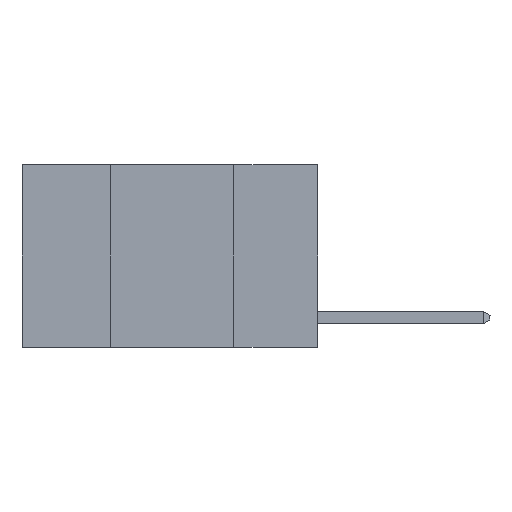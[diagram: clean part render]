
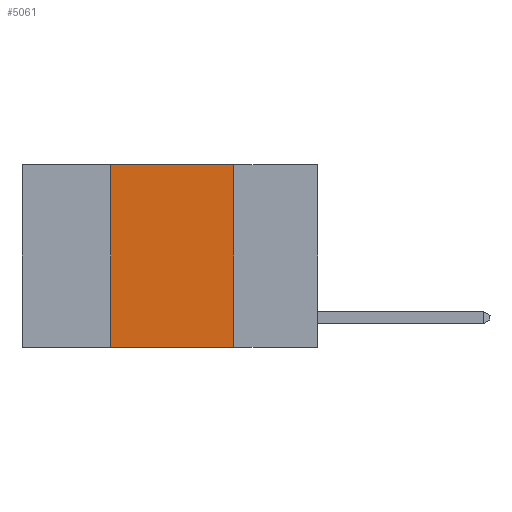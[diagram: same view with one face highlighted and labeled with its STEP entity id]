
A CAD part, left-side view. The second image highlights one B-rep face of the part: STEP entity #5061.
In plain terms, the highlighted planar face has unit normal (-1, 0, 0).
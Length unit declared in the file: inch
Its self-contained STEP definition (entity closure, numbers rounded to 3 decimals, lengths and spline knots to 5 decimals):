
#103 = ORIENTED_EDGE ( 'NONE', *, *, #5958, .F. ) ;
#251 = CARTESIAN_POINT ( 'NONE',  ( 0., 0.42, 0. ) ) ;
#466 = CARTESIAN_POINT ( 'NONE',  ( 0., 0.17, 0. ) ) ;
#514 = EDGE_LOOP ( 'NONE', ( #103, #3290, #4762, #8786 ) ) ;
#529 = EDGE_CURVE ( 'NONE', #6634, #3813, #790, .T. ) ;
#790 = LINE ( 'NONE', #2939, #5720 ) ;
#1000 = CARTESIAN_POINT ( 'NONE',  ( 0., 0.17, 0. ) ) ;
#2149 = LINE ( 'NONE', #8545, #6461 ) ;
#2500 = VERTEX_POINT ( 'NONE', #3607 ) ;
#2772 = CARTESIAN_POINT ( 'NONE',  ( 0., 0.42, -0.37 ) ) ;
#2939 = CARTESIAN_POINT ( 'NONE',  ( 0., 0.42, 0. ) ) ;
#3290 = ORIENTED_EDGE ( 'NONE', *, *, #6946, .F. ) ;
#3315 = VECTOR ( 'NONE', #8632, 39.37008 ) ;
#3607 = CARTESIAN_POINT ( 'NONE',  ( 0., 0.17, -0.37 ) ) ;
#3813 = VERTEX_POINT ( 'NONE', #251 ) ;
#3992 = DIRECTION ( 'NONE',  ( 1., 0., 0. ) ) ;
#4487 = VECTOR ( 'NONE', #8767, 39.37008 ) ;
#4660 = PLANE ( 'NONE',  #7479 ) ;
#4762 = ORIENTED_EDGE ( 'NONE', *, *, #529, .F. ) ;
#4980 = DIRECTION ( 'NONE',  ( 0., -1., 0. ) ) ;
#5061 = ADVANCED_FACE ( 'NONE', ( #8192 ), #4660, .F. ) ;
#5209 = DIRECTION ( 'NONE',  ( 0., 0., 1. ) ) ;
#5419 = DIRECTION ( 'NONE',  ( 0., 0., -1. ) ) ;
#5714 = VERTEX_POINT ( 'NONE', #466 ) ;
#5720 = VECTOR ( 'NONE', #5209, 39.37008 ) ;
#5836 = CARTESIAN_POINT ( 'NONE',  ( 0., 0.6, -0.37 ) ) ;
#5842 = EDGE_CURVE ( 'NONE', #6634, #2500, #8689, .T. ) ;
#5958 = EDGE_CURVE ( 'NONE', #5714, #2500, #7366, .T. ) ;
#6461 = VECTOR ( 'NONE', #4980, 39.37008 ) ;
#6634 = VERTEX_POINT ( 'NONE', #2772 ) ;
#6946 = EDGE_CURVE ( 'NONE', #3813, #5714, #2149, .T. ) ;
#7366 = LINE ( 'NONE', #1000, #4487 ) ;
#7479 = AXIS2_PLACEMENT_3D ( 'NONE', #7517, #3992, #5419 ) ;
#7517 = CARTESIAN_POINT ( 'NONE',  ( 0., 0.6, 0. ) ) ;
#8192 = FACE_OUTER_BOUND ( 'NONE', #514, .T. ) ;
#8545 = CARTESIAN_POINT ( 'NONE',  ( 0., 0.6, 0. ) ) ;
#8632 = DIRECTION ( 'NONE',  ( 0., -1., 0. ) ) ;
#8689 = LINE ( 'NONE', #5836, #3315 ) ;
#8767 = DIRECTION ( 'NONE',  ( 0., 0., -1. ) ) ;
#8786 = ORIENTED_EDGE ( 'NONE', *, *, #5842, .T. ) ;
